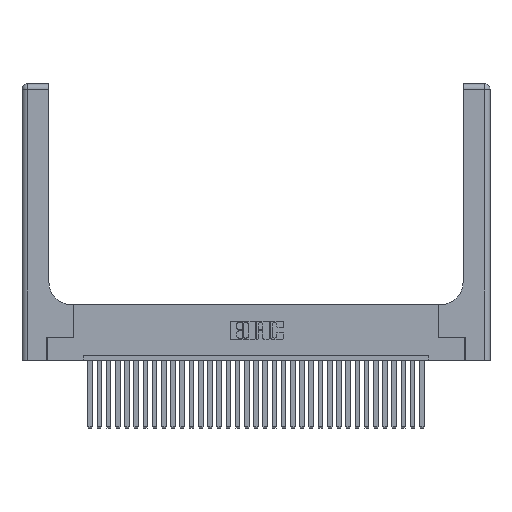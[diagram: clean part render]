
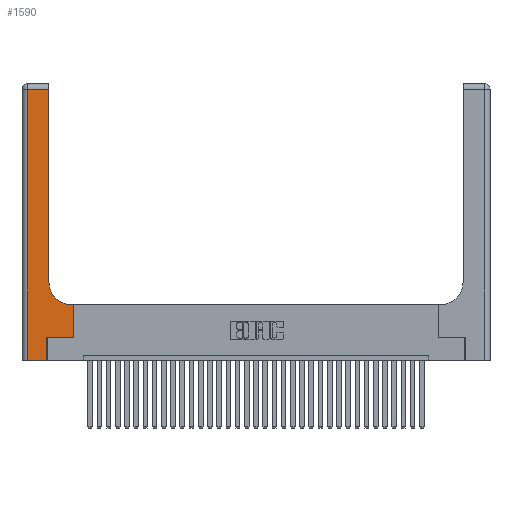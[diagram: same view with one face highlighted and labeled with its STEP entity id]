
A CAD part, top view. The second image highlights one B-rep face of the part: STEP entity #1590.
In plain terms, the highlighted planar face has unit normal (0, 0, 1).
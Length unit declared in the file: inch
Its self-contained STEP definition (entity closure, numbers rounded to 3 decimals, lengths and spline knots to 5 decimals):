
#12 = CARTESIAN_POINT ( 'NONE',  ( 0.2915, 2.94, 0.37 ) ) ;
#289 = AXIS2_PLACEMENT_3D ( 'NONE', #26254, #557, #23644 ) ;
#350 = VERTEX_POINT ( 'NONE', #1349 ) ;
#557 = DIRECTION ( 'NONE',  ( 0., 0., -1. ) ) ;
#1349 = CARTESIAN_POINT ( 'NONE',  ( 0.5585, 0.6, 0.37 ) ) ;
#1590 = ADVANCED_FACE ( 'NONE', ( #21275 ), #31432, .F. ) ;
#1625 = EDGE_CURVE ( 'NONE', #8451, #27184, #13980, .T. ) ;
#1709 = EDGE_CURVE ( 'NONE', #10881, #21457, #8315, .T. ) ;
#2113 = VECTOR ( 'NONE', #4367, 39.37008 ) ;
#3263 = DIRECTION ( 'NONE',  ( 0., -1., 0. ) ) ;
#4367 = DIRECTION ( 'NONE',  ( -1., 0., 0. ) ) ;
#5427 = DIRECTION ( 'NONE',  ( -1., 0., 0. ) ) ;
#5775 = CARTESIAN_POINT ( 'NONE',  ( 0.06, 3., 0.37 ) ) ;
#6809 = EDGE_CURVE ( 'NONE', #21457, #350, #31587, .T. ) ;
#6874 = CARTESIAN_POINT ( 'NONE',  ( 0.5415, 0.6, 0.37 ) ) ;
#7653 = ORIENTED_EDGE ( 'NONE', *, *, #1709, .T. ) ;
#7749 = VECTOR ( 'NONE', #31262, 39.37008 ) ;
#8061 = DIRECTION ( 'NONE',  ( -1., 0., 0. ) ) ;
#8224 = DIRECTION ( 'NONE',  ( 0., 1., 0. ) ) ;
#8287 = DIRECTION ( 'NONE',  ( 1., 0., 0. ) ) ;
#8315 = LINE ( 'NONE', #19250, #20041 ) ;
#8451 = VERTEX_POINT ( 'NONE', #6874 ) ;
#9577 = VERTEX_POINT ( 'NONE', #12563 ) ;
#10881 = VERTEX_POINT ( 'NONE', #32477 ) ;
#11105 = DIRECTION ( 'NONE',  ( 1., 0., 0. ) ) ;
#11154 = VERTEX_POINT ( 'NONE', #12 ) ;
#11176 = LINE ( 'NONE', #23723, #23722 ) ;
#11224 = CARTESIAN_POINT ( 'NONE',  ( 0., 0., 0.37 ) ) ;
#11330 = EDGE_CURVE ( 'NONE', #14728, #9577, #30032, .T. ) ;
#11502 = EDGE_CURVE ( 'NONE', #350, #8451, #21561, .T. ) ;
#11711 = LINE ( 'NONE', #33068, #25013 ) ;
#12504 = LINE ( 'NONE', #5775, #31493 ) ;
#12563 = CARTESIAN_POINT ( 'NONE',  ( 0.269, 0., 0.37 ) ) ;
#13152 = EDGE_CURVE ( 'NONE', #25061, #14728, #12504, .T. ) ;
#13216 = CARTESIAN_POINT ( 'NONE',  ( 0.5585, 0.25, 0.37 ) ) ;
#13277 = ORIENTED_EDGE ( 'NONE', *, *, #1625, .T. ) ;
#13980 = CIRCLE ( 'NONE', #289, 0.25 ) ;
#14659 = EDGE_CURVE ( 'NONE', #27184, #11154, #11176, .T. ) ;
#14728 = VERTEX_POINT ( 'NONE', #26647 ) ;
#16323 = ORIENTED_EDGE ( 'NONE', *, *, #6809, .T. ) ;
#19250 = CARTESIAN_POINT ( 'NONE',  ( 0.269, 0.25, 0.37 ) ) ;
#19810 = CARTESIAN_POINT ( 'NONE',  ( 0.2915, 0.6, 0.37 ) ) ;
#20041 = VECTOR ( 'NONE', #11105, 39.37008 ) ;
#20741 = ORIENTED_EDGE ( 'NONE', *, *, #13152, .T. ) ;
#20869 = CARTESIAN_POINT ( 'NONE',  ( 0., 2.94, 0.37 ) ) ;
#21038 = CARTESIAN_POINT ( 'NONE',  ( 0.2915, 0.85, 0.37 ) ) ;
#21190 = VECTOR ( 'NONE', #8287, 39.37008 ) ;
#21275 = FACE_OUTER_BOUND ( 'NONE', #23867, .T. ) ;
#21457 = VERTEX_POINT ( 'NONE', #28251 ) ;
#21561 = LINE ( 'NONE', #19810, #2113 ) ;
#23644 = DIRECTION ( 'NONE',  ( 1., 0., 0. ) ) ;
#23722 = VECTOR ( 'NONE', #8224, 39.37008 ) ;
#23723 = CARTESIAN_POINT ( 'NONE',  ( 0.2915, 3., 0.37 ) ) ;
#23759 = CARTESIAN_POINT ( 'NONE',  ( 0., 3., 0.37 ) ) ;
#23867 = EDGE_LOOP ( 'NONE', ( #28550, #24946, #20741, #31071, #32955, #7653, #16323, #25472, #13277 ) ) ;
#24946 = ORIENTED_EDGE ( 'NONE', *, *, #31534, .T. ) ;
#25013 = VECTOR ( 'NONE', #27979, 39.37008 ) ;
#25061 = VERTEX_POINT ( 'NONE', #31831 ) ;
#25472 = ORIENTED_EDGE ( 'NONE', *, *, #11502, .T. ) ;
#26237 = VECTOR ( 'NONE', #8061, 39.37008 ) ;
#26254 = CARTESIAN_POINT ( 'NONE',  ( 0.5415, 0.85, 0.37 ) ) ;
#26647 = CARTESIAN_POINT ( 'NONE',  ( 0.06, 0., 0.37 ) ) ;
#27184 = VERTEX_POINT ( 'NONE', #21038 ) ;
#27588 = EDGE_CURVE ( 'NONE', #9577, #10881, #11711, .T. ) ;
#27979 = DIRECTION ( 'NONE',  ( 0., 1., 0. ) ) ;
#28251 = CARTESIAN_POINT ( 'NONE',  ( 0.5585, 0.25, 0.37 ) ) ;
#28550 = ORIENTED_EDGE ( 'NONE', *, *, #14659, .T. ) ;
#28944 = DIRECTION ( 'NONE',  ( 0., 0., -1. ) ) ;
#29757 = AXIS2_PLACEMENT_3D ( 'NONE', #23759, #28944, #5427 ) ;
#30032 = LINE ( 'NONE', #11224, #21190 ) ;
#31071 = ORIENTED_EDGE ( 'NONE', *, *, #11330, .T. ) ;
#31262 = DIRECTION ( 'NONE',  ( 0., 1., 0. ) ) ;
#31432 = PLANE ( 'NONE',  #29757 ) ;
#31493 = VECTOR ( 'NONE', #3263, 39.37008 ) ;
#31534 = EDGE_CURVE ( 'NONE', #11154, #25061, #32700, .T. ) ;
#31587 = LINE ( 'NONE', #13216, #7749 ) ;
#31831 = CARTESIAN_POINT ( 'NONE',  ( 0.06, 2.94, 0.37 ) ) ;
#32477 = CARTESIAN_POINT ( 'NONE',  ( 0.269, 0.25, 0.37 ) ) ;
#32700 = LINE ( 'NONE', #20869, #26237 ) ;
#32955 = ORIENTED_EDGE ( 'NONE', *, *, #27588, .T. ) ;
#33068 = CARTESIAN_POINT ( 'NONE',  ( 0.269, 0., 0.37 ) ) ;
